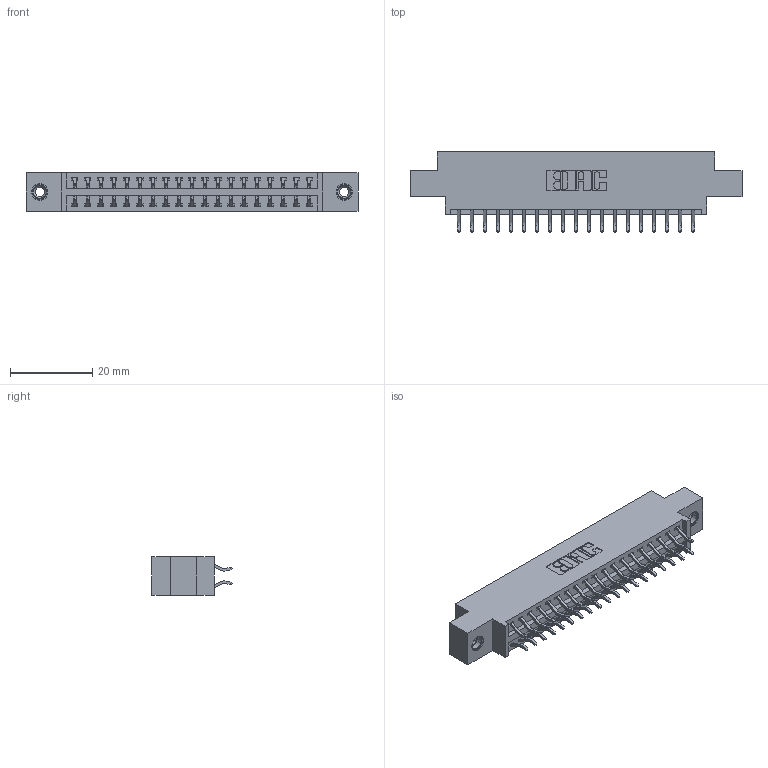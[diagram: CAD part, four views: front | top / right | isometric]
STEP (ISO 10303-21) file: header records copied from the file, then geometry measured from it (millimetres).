
FILE_DESCRIPTION (( 'STEP AP203' ), '1' );
FILE_NAME ('346-038-556-808.STEP', '2022-05-20T00:20:49', ( '' ), ( '' ), 'SwSTEP 2.0', 'SolidWorks 2020', '' );
FILE_SCHEMA (( 'CONFIG_CONTROL_DESIGN' ));
Length unit declared in the file: inch
Products named in the file (4): 345-292-001_556 Tail; 346-038-556-808; 346 Part_0.170 Offset - 0.156 Dia-TI; 345-250-001_345-250-003-102
Assembly tree (41 placements, depth 2):
  346-038-556-808
    346 Part_0.170 Offset - 0.156 Dia-TI
    345-292-001_556 Tail  x38
    345-250-001_345-250-003-102  x2
Bounding box: 80.9 x 19.57 x 9.4 mm (x, y, z)
Volume: 7547.4 mm3; surface area: 10177.2 mm2
Topology: 41 solids, 41 shells, 2390 faces, 7051 edges, 4642 vertices
Faces by surface type: plane 1594, cylinder 780, cone 12, torus 4
Entity records: 17034 total; most frequent: CARTESIAN_POINT 2839, ORIENTED_EDGE 2754, DIRECTION 2567, EDGE_CURVE 1377, VECTOR 1141, LINE 1141, VERTEX_POINT 912, AXIS2_PLACEMENT_3D 713
